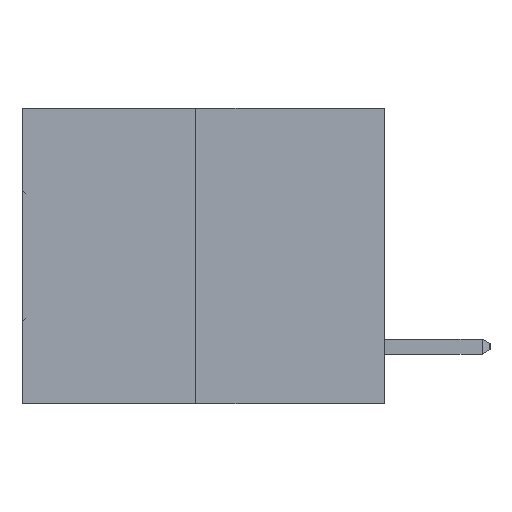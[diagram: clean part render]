
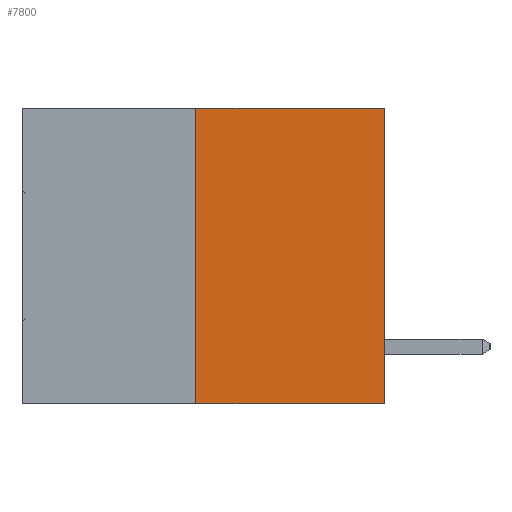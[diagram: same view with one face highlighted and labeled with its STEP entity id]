
A CAD part, left-side view. The second image highlights one B-rep face of the part: STEP entity #7800.
In plain terms, the highlighted planar face has unit normal (-1, 0, 0).
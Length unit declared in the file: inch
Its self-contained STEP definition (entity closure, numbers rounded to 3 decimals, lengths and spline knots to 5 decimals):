
#450 = ORIENTED_EDGE ( 'NONE', *, *, #4405, .T. ) ;
#1025 = LINE ( 'NONE', #7728, #2734 ) ;
#2497 = VERTEX_POINT ( 'NONE', #10055 ) ;
#2734 = VECTOR ( 'NONE', #29432, 39.37008 ) ;
#3351 = VERTEX_POINT ( 'NONE', #26561 ) ;
#4062 = ORIENTED_EDGE ( 'NONE', *, *, #22641, .T. ) ;
#4331 = VECTOR ( 'NONE', #4758, 39.37008 ) ;
#4405 = EDGE_CURVE ( 'NONE', #2497, #26178, #22921, .T. ) ;
#4758 = DIRECTION ( 'NONE',  ( 0., 0., 1. ) ) ;
#5291 = CARTESIAN_POINT ( 'NONE',  ( 0., 0.312, 0. ) ) ;
#5767 = CARTESIAN_POINT ( 'NONE',  ( 0., 0.6, 0. ) ) ;
#6632 = CARTESIAN_POINT ( 'NONE',  ( 0., 0.6, 0. ) ) ;
#6654 = VECTOR ( 'NONE', #26945, 39.37008 ) ;
#7728 = CARTESIAN_POINT ( 'NONE',  ( 0., 0.312, -0.49 ) ) ;
#7731 = CARTESIAN_POINT ( 'NONE',  ( 0., 0.6, -0.49 ) ) ;
#7800 = ADVANCED_FACE ( 'NONE', ( #31266 ), #19273, .F. ) ;
#10055 = CARTESIAN_POINT ( 'NONE',  ( 0., 0., -0.49 ) ) ;
#10833 = DIRECTION ( 'NONE',  ( 0., 0., -1. ) ) ;
#14662 = EDGE_LOOP ( 'NONE', ( #27432, #4062, #450, #27233 ) ) ;
#16704 = EDGE_CURVE ( 'NONE', #34686, #26178, #29645, .T. ) ;
#18728 = EDGE_CURVE ( 'NONE', #3351, #34686, #1025, .T. ) ;
#19153 = DIRECTION ( 'NONE',  ( 1., 0., 0. ) ) ;
#19229 = AXIS2_PLACEMENT_3D ( 'NONE', #5767, #19153, #10833 ) ;
#19273 = PLANE ( 'NONE',  #19229 ) ;
#21052 = LINE ( 'NONE', #7731, #6654 ) ;
#21380 = CARTESIAN_POINT ( 'NONE',  ( 0., 0., 0. ) ) ;
#22641 = EDGE_CURVE ( 'NONE', #3351, #2497, #21052, .T. ) ;
#22921 = LINE ( 'NONE', #34127, #4331 ) ;
#23674 = VECTOR ( 'NONE', #33646, 39.37008 ) ;
#26178 = VERTEX_POINT ( 'NONE', #21380 ) ;
#26561 = CARTESIAN_POINT ( 'NONE',  ( 0., 0.312, -0.49 ) ) ;
#26945 = DIRECTION ( 'NONE',  ( 0., -1., 0. ) ) ;
#27233 = ORIENTED_EDGE ( 'NONE', *, *, #16704, .F. ) ;
#27432 = ORIENTED_EDGE ( 'NONE', *, *, #18728, .F. ) ;
#29432 = DIRECTION ( 'NONE',  ( 0., 0., 1. ) ) ;
#29645 = LINE ( 'NONE', #6632, #23674 ) ;
#31266 = FACE_OUTER_BOUND ( 'NONE', #14662, .T. ) ;
#33646 = DIRECTION ( 'NONE',  ( 0., -1., 0. ) ) ;
#34127 = CARTESIAN_POINT ( 'NONE',  ( 0., 0., 0. ) ) ;
#34686 = VERTEX_POINT ( 'NONE', #5291 ) ;
